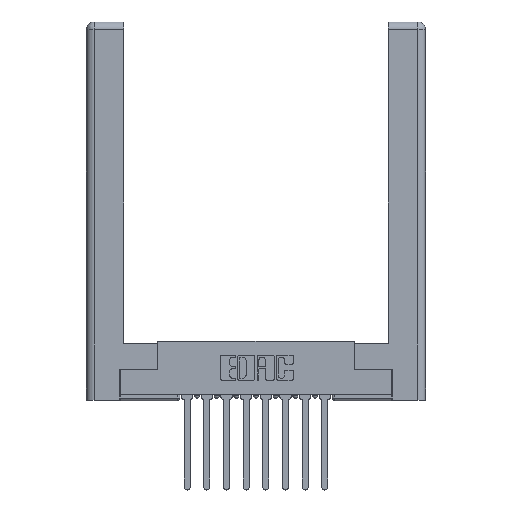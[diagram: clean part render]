
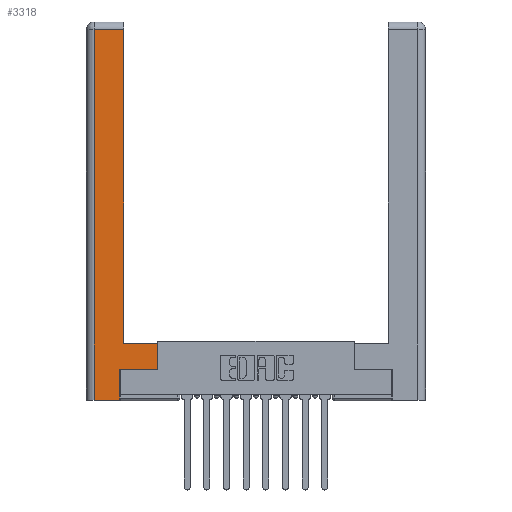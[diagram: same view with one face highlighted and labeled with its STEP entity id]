
A CAD part, top view. The second image highlights one B-rep face of the part: STEP entity #3318.
In plain terms, the highlighted planar face has unit normal (0, 0, 1).
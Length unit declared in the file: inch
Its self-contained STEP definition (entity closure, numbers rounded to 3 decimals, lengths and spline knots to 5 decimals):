
#216 = DIRECTION ( 'NONE',  ( 1., 0., 0. ) ) ;
#352 = CARTESIAN_POINT ( 'NONE',  ( 0.265, 0.245, 0. ) ) ;
#403 = ORIENTED_EDGE ( 'NONE', *, *, #3462, .T. ) ;
#420 = VECTOR ( 'NONE', #2760, 39.37008 ) ;
#657 = CARTESIAN_POINT ( 'NONE',  ( 0.565, 0.45, 0. ) ) ;
#1219 = CARTESIAN_POINT ( 'NONE',  ( 0.565, 0.245, 0. ) ) ;
#1271 = DIRECTION ( 'NONE',  ( -1., 0., 0. ) ) ;
#1415 = PLANE ( 'NONE',  #6413 ) ;
#1692 = DIRECTION ( 'NONE',  ( 0., 1., 0. ) ) ;
#1804 = CARTESIAN_POINT ( 'NONE',  ( 0.265, 0., 0. ) ) ;
#2385 = LINE ( 'NONE', #7642, #9604 ) ;
#2440 = VERTEX_POINT ( 'NONE', #1804 ) ;
#2613 = LINE ( 'NONE', #13604, #6631 ) ;
#2737 = VERTEX_POINT ( 'NONE', #8468 ) ;
#2760 = DIRECTION ( 'NONE',  ( 1., 0., 0. ) ) ;
#2976 = LINE ( 'NONE', #8432, #12495 ) ;
#3318 = ADVANCED_FACE ( 'NONE', ( #13112 ), #1415, .F. ) ;
#3328 = DIRECTION ( 'NONE',  ( 0., 0., -1. ) ) ;
#3360 = VERTEX_POINT ( 'NONE', #9972 ) ;
#3462 = EDGE_CURVE ( 'NONE', #6053, #3360, #2613, .T. ) ;
#3600 = DIRECTION ( 'NONE',  ( -1., 0., 0. ) ) ;
#3666 = EDGE_CURVE ( 'NONE', #2440, #10070, #2976, .T. ) ;
#4090 = EDGE_CURVE ( 'NONE', #2737, #11402, #8662, .T. ) ;
#4117 = VERTEX_POINT ( 'NONE', #6295 ) ;
#4251 = LINE ( 'NONE', #1219, #6799 ) ;
#4534 = CARTESIAN_POINT ( 'NONE',  ( 0.295, 2.94, 0. ) ) ;
#4779 = LINE ( 'NONE', #13381, #9144 ) ;
#5021 = EDGE_CURVE ( 'NONE', #11323, #2737, #2385, .T. ) ;
#5645 = EDGE_LOOP ( 'NONE', ( #5679, #11731, #11593, #8727, #12150, #10814, #13473, #403 ) ) ;
#5679 = ORIENTED_EDGE ( 'NONE', *, *, #6497, .T. ) ;
#5999 = CARTESIAN_POINT ( 'NONE',  ( 0.0615, 0., 0. ) ) ;
#6053 = VERTEX_POINT ( 'NONE', #657 ) ;
#6118 = EDGE_CURVE ( 'NONE', #11402, #2440, #13469, .T. ) ;
#6295 = CARTESIAN_POINT ( 'NONE',  ( 0.565, 0.245, 0. ) ) ;
#6413 = AXIS2_PLACEMENT_3D ( 'NONE', #11047, #3328, #3600 ) ;
#6431 = DIRECTION ( 'NONE',  ( 0., -1., 0. ) ) ;
#6497 = EDGE_CURVE ( 'NONE', #3360, #11323, #4779, .T. ) ;
#6631 = VECTOR ( 'NONE', #6885, 39.37008 ) ;
#6799 = VECTOR ( 'NONE', #216, 39.37008 ) ;
#6885 = DIRECTION ( 'NONE',  ( -1., 0., 0. ) ) ;
#7236 = DIRECTION ( 'NONE',  ( 0., 1., 0. ) ) ;
#7642 = CARTESIAN_POINT ( 'NONE',  ( 0.0615, 2.94, 0. ) ) ;
#8014 = CARTESIAN_POINT ( 'NONE',  ( 0.265, 0., 0. ) ) ;
#8432 = CARTESIAN_POINT ( 'NONE',  ( 0.265, 0.245, 0. ) ) ;
#8468 = CARTESIAN_POINT ( 'NONE',  ( 0.0615, 2.94, 0. ) ) ;
#8662 = LINE ( 'NONE', #11784, #13432 ) ;
#8727 = ORIENTED_EDGE ( 'NONE', *, *, #6118, .T. ) ;
#9144 = VECTOR ( 'NONE', #1692, 39.37008 ) ;
#9365 = DIRECTION ( 'NONE',  ( 0., 1., 0. ) ) ;
#9604 = VECTOR ( 'NONE', #1271, 39.37008 ) ;
#9972 = CARTESIAN_POINT ( 'NONE',  ( 0.295, 0.45, 0. ) ) ;
#10070 = VERTEX_POINT ( 'NONE', #352 ) ;
#10360 = CARTESIAN_POINT ( 'NONE',  ( 0.565, 0.45, 0. ) ) ;
#10814 = ORIENTED_EDGE ( 'NONE', *, *, #12909, .T. ) ;
#11047 = CARTESIAN_POINT ( 'NONE',  ( 0., 0., 0. ) ) ;
#11323 = VERTEX_POINT ( 'NONE', #4534 ) ;
#11402 = VERTEX_POINT ( 'NONE', #5999 ) ;
#11441 = EDGE_CURVE ( 'NONE', #4117, #6053, #11494, .T. ) ;
#11494 = LINE ( 'NONE', #10360, #12484 ) ;
#11593 = ORIENTED_EDGE ( 'NONE', *, *, #4090, .T. ) ;
#11731 = ORIENTED_EDGE ( 'NONE', *, *, #5021, .T. ) ;
#11784 = CARTESIAN_POINT ( 'NONE',  ( 0.0615, 0., 0. ) ) ;
#12150 = ORIENTED_EDGE ( 'NONE', *, *, #3666, .T. ) ;
#12484 = VECTOR ( 'NONE', #9365, 39.37008 ) ;
#12495 = VECTOR ( 'NONE', #7236, 39.37008 ) ;
#12909 = EDGE_CURVE ( 'NONE', #10070, #4117, #4251, .T. ) ;
#13112 = FACE_OUTER_BOUND ( 'NONE', #5645, .T. ) ;
#13381 = CARTESIAN_POINT ( 'NONE',  ( 0.295, 3., 0. ) ) ;
#13432 = VECTOR ( 'NONE', #6431, 39.37008 ) ;
#13469 = LINE ( 'NONE', #8014, #420 ) ;
#13473 = ORIENTED_EDGE ( 'NONE', *, *, #11441, .T. ) ;
#13604 = CARTESIAN_POINT ( 'NONE',  ( 0.295, 0.45, 0. ) ) ;
